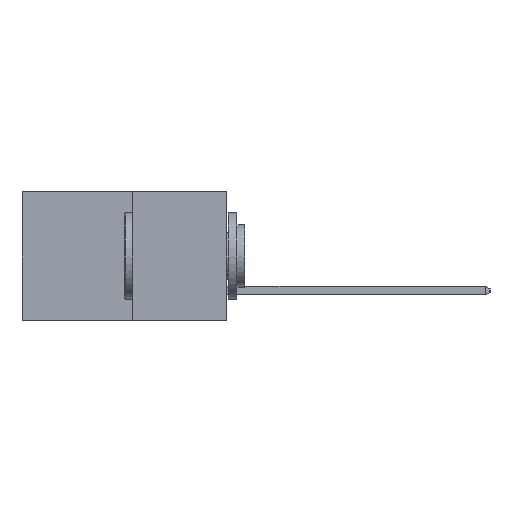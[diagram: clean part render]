
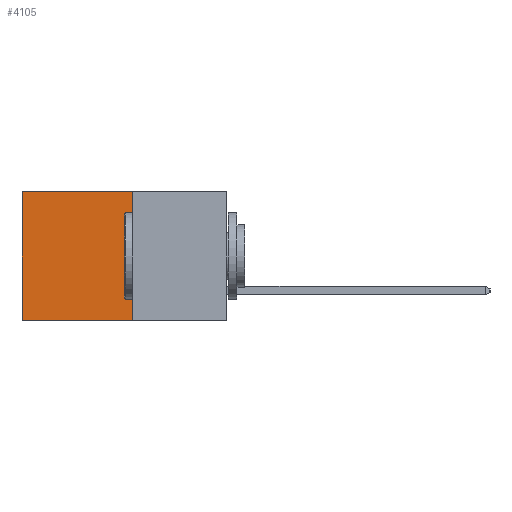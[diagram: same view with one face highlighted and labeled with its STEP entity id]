
A CAD part, left-side view. The second image highlights one B-rep face of the part: STEP entity #4105.
In plain terms, the highlighted planar face has unit normal (-1, 0, 0).
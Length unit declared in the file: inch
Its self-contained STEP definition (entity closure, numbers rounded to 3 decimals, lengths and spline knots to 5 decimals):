
#57 = VECTOR ( 'NONE', #4263, 39.37008 ) ;
#178 = CARTESIAN_POINT ( 'NONE',  ( 0.277, 0.27, 0. ) ) ;
#861 = VERTEX_POINT ( 'NONE', #6892 ) ;
#1001 = EDGE_CURVE ( 'NONE', #1142, #5578, #5374, .T. ) ;
#1045 = EDGE_CURVE ( 'NONE', #5578, #5385, #4995, .T. ) ;
#1142 = VERTEX_POINT ( 'NONE', #178 ) ;
#1624 = AXIS2_PLACEMENT_3D ( 'NONE', #5214, #5431, #3840 ) ;
#1987 = LINE ( 'NONE', #5363, #6918 ) ;
#2688 = FACE_OUTER_BOUND ( 'NONE', #2885, .T. ) ;
#2885 = EDGE_LOOP ( 'NONE', ( #7890, #4724, #4763, #6380 ) ) ;
#3791 = CARTESIAN_POINT ( 'NONE',  ( 0.277, 0.59, -0.37 ) ) ;
#3840 = DIRECTION ( 'NONE',  ( 0., 0., -1. ) ) ;
#3994 = EDGE_CURVE ( 'NONE', #1142, #861, #1987, .T. ) ;
#4005 = EDGE_CURVE ( 'NONE', #861, #5385, #6704, .T. ) ;
#4105 = ADVANCED_FACE ( 'NONE', ( #2688 ), #8049, .F. ) ;
#4263 = DIRECTION ( 'NONE',  ( 0., 0., -1. ) ) ;
#4662 = CARTESIAN_POINT ( 'NONE',  ( 0.277, 0.27, -0.37 ) ) ;
#4724 = ORIENTED_EDGE ( 'NONE', *, *, #1045, .F. ) ;
#4763 = ORIENTED_EDGE ( 'NONE', *, *, #1001, .F. ) ;
#4995 = LINE ( 'NONE', #5974, #6417 ) ;
#5214 = CARTESIAN_POINT ( 'NONE',  ( 0.277, 0.27, -0.37 ) ) ;
#5363 = CARTESIAN_POINT ( 'NONE',  ( 0.277, 0.27, 0. ) ) ;
#5374 = LINE ( 'NONE', #6977, #6802 ) ;
#5385 = VERTEX_POINT ( 'NONE', #7298 ) ;
#5431 = DIRECTION ( 'NONE',  ( 1., 0., 0. ) ) ;
#5578 = VERTEX_POINT ( 'NONE', #4662 ) ;
#5784 = DIRECTION ( 'NONE',  ( 0., 1., 0. ) ) ;
#5974 = CARTESIAN_POINT ( 'NONE',  ( 0.277, 0.27, -0.37 ) ) ;
#6380 = ORIENTED_EDGE ( 'NONE', *, *, #3994, .T. ) ;
#6417 = VECTOR ( 'NONE', #5784, 39.37008 ) ;
#6704 = LINE ( 'NONE', #3791, #57 ) ;
#6802 = VECTOR ( 'NONE', #6931, 39.37008 ) ;
#6892 = CARTESIAN_POINT ( 'NONE',  ( 0.277, 0.59, 0. ) ) ;
#6918 = VECTOR ( 'NONE', #7154, 39.37008 ) ;
#6931 = DIRECTION ( 'NONE',  ( 0., 0., -1. ) ) ;
#6977 = CARTESIAN_POINT ( 'NONE',  ( 0.277, 0.27, -0.37 ) ) ;
#7154 = DIRECTION ( 'NONE',  ( 0., 1., 0. ) ) ;
#7298 = CARTESIAN_POINT ( 'NONE',  ( 0.277, 0.59, -0.37 ) ) ;
#7890 = ORIENTED_EDGE ( 'NONE', *, *, #4005, .T. ) ;
#8049 = PLANE ( 'NONE',  #1624 ) ;
